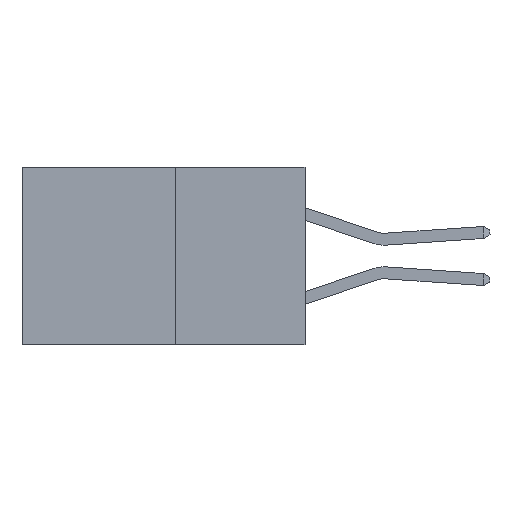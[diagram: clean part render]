
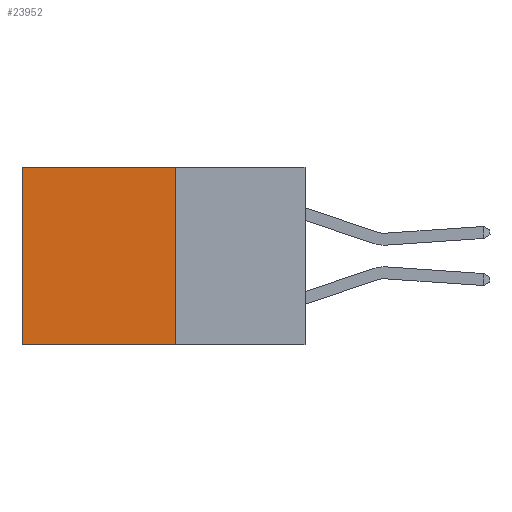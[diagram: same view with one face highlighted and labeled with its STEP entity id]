
A CAD part, left-side view. The second image highlights one B-rep face of the part: STEP entity #23952.
In plain terms, the highlighted planar face has unit normal (-1, 0, 0).
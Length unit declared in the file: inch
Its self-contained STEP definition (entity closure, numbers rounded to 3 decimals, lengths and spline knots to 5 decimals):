
#4136 = LINE ( 'NONE', #8187, #10459 ) ;
#5216 = ORIENTED_EDGE ( 'NONE', *, *, #9733, .F. ) ;
#5367 = DIRECTION ( 'NONE',  ( 1., 0., 0. ) ) ;
#5844 = ORIENTED_EDGE ( 'NONE', *, *, #32886, .T. ) ;
#6300 = CARTESIAN_POINT ( 'NONE',  ( 0.277, 0.27, 0. ) ) ;
#8187 = CARTESIAN_POINT ( 'NONE',  ( 0.277, 0.27, -0.37 ) ) ;
#8445 = CARTESIAN_POINT ( 'NONE',  ( 0.277, 0.59, 0. ) ) ;
#9733 = EDGE_CURVE ( 'NONE', #18419, #27120, #20081, .T. ) ;
#10459 = VECTOR ( 'NONE', #31883, 39.37008 ) ;
#11617 = CARTESIAN_POINT ( 'NONE',  ( 0.277, 0.27, -0.37 ) ) ;
#11644 = CARTESIAN_POINT ( 'NONE',  ( 0.277, 0.59, -0.37 ) ) ;
#12283 = VECTOR ( 'NONE', #30876, 39.37008 ) ;
#13248 = LINE ( 'NONE', #29943, #34113 ) ;
#13569 = FACE_OUTER_BOUND ( 'NONE', #27735, .T. ) ;
#13608 = ORIENTED_EDGE ( 'NONE', *, *, #30285, .F. ) ;
#14239 = DIRECTION ( 'NONE',  ( 0., 0., -1. ) ) ;
#14379 = DIRECTION ( 'NONE',  ( 0., 1., 0. ) ) ;
#17308 = LINE ( 'NONE', #6300, #22628 ) ;
#18313 = VERTEX_POINT ( 'NONE', #8445 ) ;
#18419 = VERTEX_POINT ( 'NONE', #11617 ) ;
#18466 = ORIENTED_EDGE ( 'NONE', *, *, #28420, .T. ) ;
#20081 = LINE ( 'NONE', #28277, #12283 ) ;
#21263 = CARTESIAN_POINT ( 'NONE',  ( 0.277, 0.27, -0.37 ) ) ;
#21719 = AXIS2_PLACEMENT_3D ( 'NONE', #21263, #5367, #23921 ) ;
#22628 = VECTOR ( 'NONE', #14379, 39.37008 ) ;
#23921 = DIRECTION ( 'NONE',  ( 0., 0., -1. ) ) ;
#23952 = ADVANCED_FACE ( 'NONE', ( #13569 ), #26433, .F. ) ;
#25694 = CARTESIAN_POINT ( 'NONE',  ( 0.277, 0.27, 0. ) ) ;
#26433 = PLANE ( 'NONE',  #21719 ) ;
#26722 = VERTEX_POINT ( 'NONE', #25694 ) ;
#27120 = VERTEX_POINT ( 'NONE', #11644 ) ;
#27735 = EDGE_LOOP ( 'NONE', ( #18466, #5216, #13608, #5844 ) ) ;
#28277 = CARTESIAN_POINT ( 'NONE',  ( 0.277, 0.27, -0.37 ) ) ;
#28420 = EDGE_CURVE ( 'NONE', #18313, #27120, #13248, .T. ) ;
#29943 = CARTESIAN_POINT ( 'NONE',  ( 0.277, 0.59, -0.37 ) ) ;
#30285 = EDGE_CURVE ( 'NONE', #26722, #18419, #4136, .T. ) ;
#30876 = DIRECTION ( 'NONE',  ( 0., 1., 0. ) ) ;
#31883 = DIRECTION ( 'NONE',  ( 0., 0., -1. ) ) ;
#32886 = EDGE_CURVE ( 'NONE', #26722, #18313, #17308, .T. ) ;
#34113 = VECTOR ( 'NONE', #14239, 39.37008 ) ;
